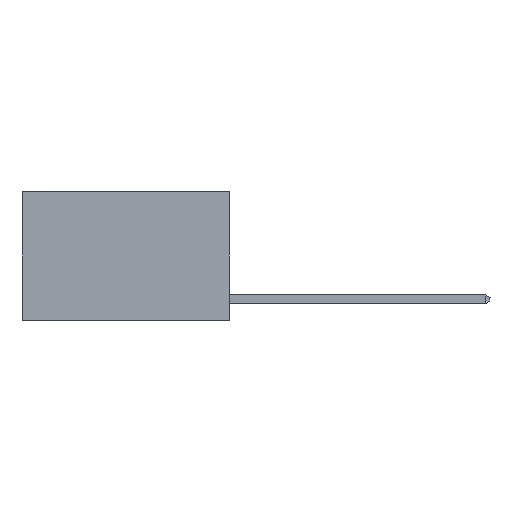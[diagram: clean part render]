
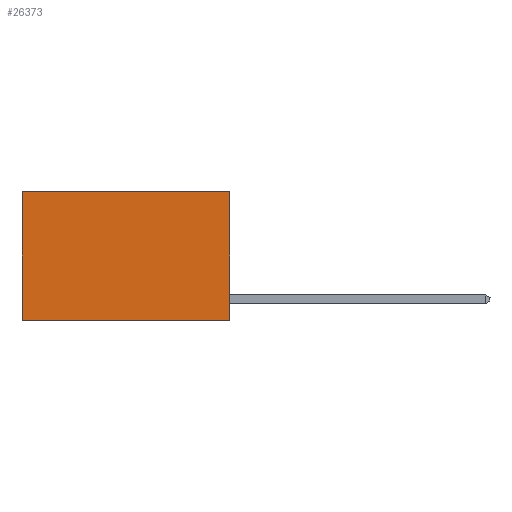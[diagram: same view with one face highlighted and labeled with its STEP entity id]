
A CAD part, left-side view. The second image highlights one B-rep face of the part: STEP entity #26373.
In plain terms, the highlighted planar face has unit normal (-1, 0, 0).
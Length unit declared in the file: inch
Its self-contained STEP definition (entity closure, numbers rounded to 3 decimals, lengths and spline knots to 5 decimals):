
#549 = DIRECTION ( 'NONE',  ( 0., 1., 0. ) ) ;
#972 = CARTESIAN_POINT ( 'NONE',  ( 0.2625, 0.6, -0.37 ) ) ;
#1430 = ORIENTED_EDGE ( 'NONE', *, *, #1609, .F. ) ;
#1609 = EDGE_CURVE ( 'NONE', #3883, #16400, #8223, .T. ) ;
#2240 = EDGE_CURVE ( 'NONE', #18921, #16400, #25036, .T. ) ;
#3883 = VERTEX_POINT ( 'NONE', #25012 ) ;
#4923 = CARTESIAN_POINT ( 'NONE',  ( 0.2625, 0., 0. ) ) ;
#6189 = DIRECTION ( 'NONE',  ( 0., 0., -1. ) ) ;
#6308 = EDGE_LOOP ( 'NONE', ( #13175, #1430, #7888, #21371 ) ) ;
#6413 = AXIS2_PLACEMENT_3D ( 'NONE', #4923, #13791, #27168 ) ;
#7386 = DIRECTION ( 'NONE',  ( 0., 0., -1. ) ) ;
#7888 = ORIENTED_EDGE ( 'NONE', *, *, #16522, .F. ) ;
#8223 = LINE ( 'NONE', #17159, #9652 ) ;
#8326 = VECTOR ( 'NONE', #549, 39.37008 ) ;
#9428 = PLANE ( 'NONE',  #6413 ) ;
#9652 = VECTOR ( 'NONE', #17588, 39.37008 ) ;
#11756 = CARTESIAN_POINT ( 'NONE',  ( 0.2625, 0.6, 0. ) ) ;
#12686 = CARTESIAN_POINT ( 'NONE',  ( 0.2625, 0., 0. ) ) ;
#13026 = CARTESIAN_POINT ( 'NONE',  ( 0.2625, 0., 0. ) ) ;
#13175 = ORIENTED_EDGE ( 'NONE', *, *, #2240, .T. ) ;
#13791 = DIRECTION ( 'NONE',  ( 1., 0., 0. ) ) ;
#14938 = LINE ( 'NONE', #13026, #23507 ) ;
#15829 = CARTESIAN_POINT ( 'NONE',  ( 0.2625, 0., 0. ) ) ;
#16400 = VERTEX_POINT ( 'NONE', #972 ) ;
#16522 = EDGE_CURVE ( 'NONE', #27269, #3883, #14938, .T. ) ;
#17159 = CARTESIAN_POINT ( 'NONE',  ( 0.2625, 0., -0.37 ) ) ;
#17555 = EDGE_CURVE ( 'NONE', #27269, #18921, #20659, .T. ) ;
#17588 = DIRECTION ( 'NONE',  ( 0., 1., 0. ) ) ;
#18580 = VECTOR ( 'NONE', #7386, 39.37008 ) ;
#18921 = VERTEX_POINT ( 'NONE', #22970 ) ;
#20659 = LINE ( 'NONE', #15829, #8326 ) ;
#21371 = ORIENTED_EDGE ( 'NONE', *, *, #17555, .T. ) ;
#22970 = CARTESIAN_POINT ( 'NONE',  ( 0.2625, 0.6, 0. ) ) ;
#23507 = VECTOR ( 'NONE', #6189, 39.37008 ) ;
#25012 = CARTESIAN_POINT ( 'NONE',  ( 0.2625, 0., -0.37 ) ) ;
#25036 = LINE ( 'NONE', #11756, #18580 ) ;
#26373 = ADVANCED_FACE ( 'NONE', ( #27031 ), #9428, .F. ) ;
#27031 = FACE_OUTER_BOUND ( 'NONE', #6308, .T. ) ;
#27168 = DIRECTION ( 'NONE',  ( 0., 0., -1. ) ) ;
#27269 = VERTEX_POINT ( 'NONE', #12686 ) ;
